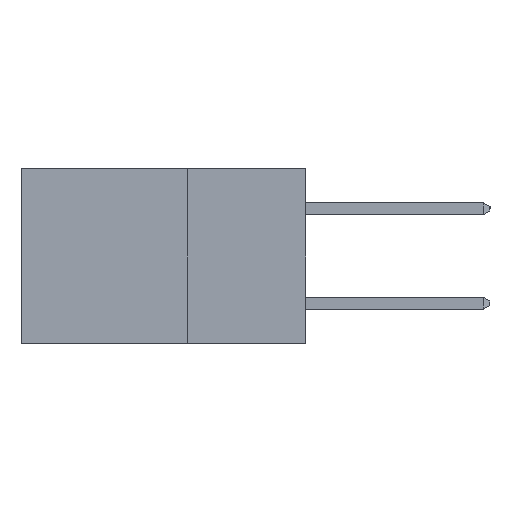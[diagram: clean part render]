
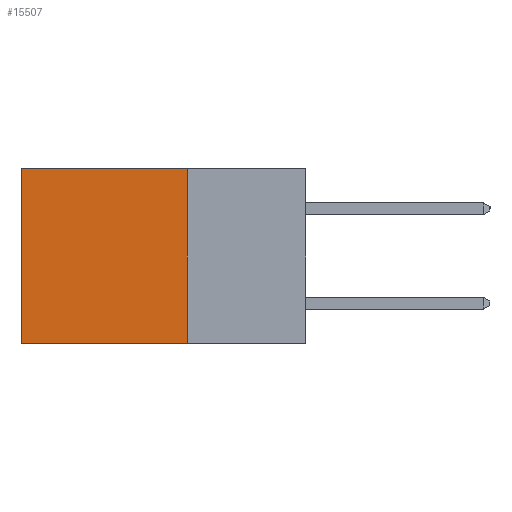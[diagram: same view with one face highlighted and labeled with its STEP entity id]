
A CAD part, left-side view. The second image highlights one B-rep face of the part: STEP entity #15507.
In plain terms, the highlighted planar face has unit normal (-1, 0, 0).
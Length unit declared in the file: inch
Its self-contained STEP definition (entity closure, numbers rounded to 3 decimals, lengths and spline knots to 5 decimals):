
#303 = CARTESIAN_POINT ( 'NONE',  ( 0.2615, 0.6, -0.37 ) ) ;
#404 = DIRECTION ( 'NONE',  ( 0., 1., 0. ) ) ;
#840 = VERTEX_POINT ( 'NONE', #18645 ) ;
#1174 = LINE ( 'NONE', #13354, #17515 ) ;
#1591 = EDGE_CURVE ( 'NONE', #840, #9194, #9637, .T. ) ;
#2899 = ORIENTED_EDGE ( 'NONE', *, *, #1591, .F. ) ;
#4077 = ORIENTED_EDGE ( 'NONE', *, *, #17773, .T. ) ;
#4275 = DIRECTION ( 'NONE',  ( 1., 0., 0. ) ) ;
#4522 = CARTESIAN_POINT ( 'NONE',  ( 0.2615, 0.6, 0. ) ) ;
#4578 = VECTOR ( 'NONE', #6506, 39.37008 ) ;
#4627 = DIRECTION ( 'NONE',  ( 0., 0., -1. ) ) ;
#5790 = PLANE ( 'NONE',  #13225 ) ;
#6506 = DIRECTION ( 'NONE',  ( 0., 0., -1. ) ) ;
#6955 = EDGE_LOOP ( 'NONE', ( #13392, #2899, #7537, #4077 ) ) ;
#7184 = CARTESIAN_POINT ( 'NONE',  ( 0.2615, 0.6, -0.37 ) ) ;
#7537 = ORIENTED_EDGE ( 'NONE', *, *, #16385, .F. ) ;
#9194 = VERTEX_POINT ( 'NONE', #7184 ) ;
#9637 = LINE ( 'NONE', #15832, #18496 ) ;
#9988 = EDGE_CURVE ( 'NONE', #17891, #9194, #11064, .T. ) ;
#10460 = DIRECTION ( 'NONE',  ( 0., 0., -1. ) ) ;
#11064 = LINE ( 'NONE', #303, #4578 ) ;
#11567 = CARTESIAN_POINT ( 'NONE',  ( 0.2615, 0.25, 0. ) ) ;
#11953 = VECTOR ( 'NONE', #4627, 39.37008 ) ;
#13225 = AXIS2_PLACEMENT_3D ( 'NONE', #18175, #4275, #10460 ) ;
#13354 = CARTESIAN_POINT ( 'NONE',  ( 0.2615, 0.25, 0. ) ) ;
#13392 = ORIENTED_EDGE ( 'NONE', *, *, #9988, .T. ) ;
#15507 = ADVANCED_FACE ( 'NONE', ( #19676 ), #5790, .F. ) ;
#15832 = CARTESIAN_POINT ( 'NONE',  ( 0.2615, 0.25, -0.37 ) ) ;
#16385 = EDGE_CURVE ( 'NONE', #18667, #840, #19835, .T. ) ;
#17515 = VECTOR ( 'NONE', #19433, 39.37008 ) ;
#17773 = EDGE_CURVE ( 'NONE', #18667, #17891, #1174, .T. ) ;
#17891 = VERTEX_POINT ( 'NONE', #4522 ) ;
#18175 = CARTESIAN_POINT ( 'NONE',  ( 0.2615, 0.25, -0.37 ) ) ;
#18496 = VECTOR ( 'NONE', #404, 39.37008 ) ;
#18519 = CARTESIAN_POINT ( 'NONE',  ( 0.2615, 0.25, -0.37 ) ) ;
#18645 = CARTESIAN_POINT ( 'NONE',  ( 0.2615, 0.25, -0.37 ) ) ;
#18667 = VERTEX_POINT ( 'NONE', #11567 ) ;
#19433 = DIRECTION ( 'NONE',  ( 0., 1., 0. ) ) ;
#19676 = FACE_OUTER_BOUND ( 'NONE', #6955, .T. ) ;
#19835 = LINE ( 'NONE', #18519, #11953 ) ;
